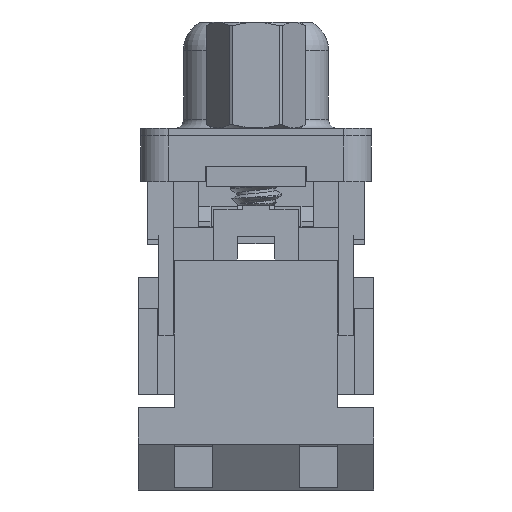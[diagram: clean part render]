
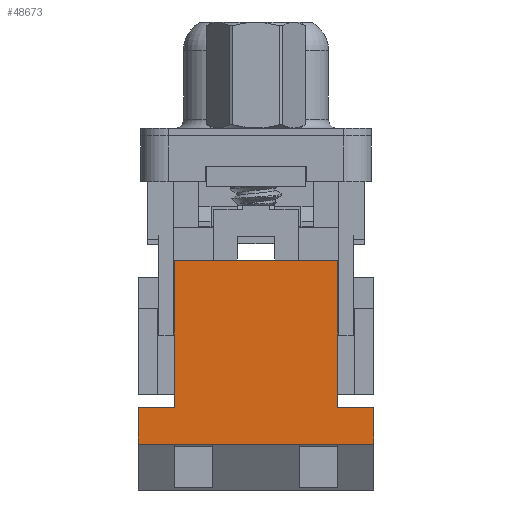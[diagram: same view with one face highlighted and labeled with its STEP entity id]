
A CAD part, left-side view. The second image highlights one B-rep face of the part: STEP entity #48673.
In plain terms, the highlighted planar face has unit normal (-1, 0, 0).
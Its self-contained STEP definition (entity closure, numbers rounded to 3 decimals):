
#1239 = EDGE_CURVE ( 'NONE', #46045, #82600, #1669, .T. ) ;
#1565 = LINE ( 'NONE', #59282, #43901 ) ;
#1669 = LINE ( 'NONE', #27736, #4810 ) ;
#4810 = VECTOR ( 'NONE', #8078, 1000. ) ;
#5013 = CARTESIAN_POINT ( 'NONE',  ( 3.245, 6.425, -14.8 ) ) ;
#7446 = ORIENTED_EDGE ( 'NONE', *, *, #13543, .F. ) ;
#7555 = DIRECTION ( 'NONE',  ( 0., -1., 0. ) ) ;
#8078 = DIRECTION ( 'NONE',  ( 0., 0., -1. ) ) ;
#9558 = EDGE_CURVE ( 'NONE', #14567, #82600, #25720, .T. ) ;
#10601 = CARTESIAN_POINT ( 'NONE',  ( 3.245, 4.45, -6.8 ) ) ;
#11469 = ORIENTED_EDGE ( 'NONE', *, *, #55813, .T. ) ;
#12076 = CARTESIAN_POINT ( 'NONE',  ( 3.245, -6.425, -16.8 ) ) ;
#13543 = EDGE_CURVE ( 'NONE', #46045, #62165, #39611, .T. ) ;
#14464 = CARTESIAN_POINT ( 'NONE',  ( 3.245, 6.425, -14.8 ) ) ;
#14567 = VERTEX_POINT ( 'NONE', #75580 ) ;
#16999 = LINE ( 'NONE', #43079, #81267 ) ;
#17155 = FACE_OUTER_BOUND ( 'NONE', #45554, .T. ) ;
#19388 = LINE ( 'NONE', #71533, #65400 ) ;
#20786 = EDGE_CURVE ( 'NONE', #35050, #14567, #19388, .T. ) ;
#21862 = PLANE ( 'NONE',  #29970 ) ;
#25720 = LINE ( 'NONE', #12076, #68399 ) ;
#27736 = CARTESIAN_POINT ( 'NONE',  ( 3.245, 6.425, -15.3 ) ) ;
#29970 = AXIS2_PLACEMENT_3D ( 'NONE', #43231, #67616, #69303 ) ;
#33811 = ORIENTED_EDGE ( 'NONE', *, *, #1239, .T. ) ;
#34139 = ORIENTED_EDGE ( 'NONE', *, *, #72278, .F. ) ;
#35050 = VERTEX_POINT ( 'NONE', #50139 ) ;
#39611 = LINE ( 'NONE', #78924, #49628 ) ;
#40540 = DIRECTION ( 'NONE',  ( 0., -1., 0. ) ) ;
#41027 = VERTEX_POINT ( 'NONE', #61676 ) ;
#41517 = CARTESIAN_POINT ( 'NONE',  ( 3.245, -4.45, -6.8 ) ) ;
#42377 = LINE ( 'NONE', #41517, #46023 ) ;
#43079 = CARTESIAN_POINT ( 'NONE',  ( 3.245, 4.45, -6.8 ) ) ;
#43231 = CARTESIAN_POINT ( 'NONE',  ( 3.245, -6.425, -15.3 ) ) ;
#43901 = VECTOR ( 'NONE', #52862, 1000. ) ;
#45554 = EDGE_LOOP ( 'NONE', ( #33811, #54687, #80344, #73086, #34139, #77305, #11469, #7446 ) ) ;
#46023 = VECTOR ( 'NONE', #67600, 1000. ) ;
#46045 = VERTEX_POINT ( 'NONE', #5013 ) ;
#48509 = VERTEX_POINT ( 'NONE', #73592 ) ;
#48673 = ADVANCED_FACE ( 'NONE', ( #17155 ), #21862, .F. ) ;
#49628 = VECTOR ( 'NONE', #7555, 1000. ) ;
#50139 = CARTESIAN_POINT ( 'NONE',  ( 3.245, -6.425, -14.8 ) ) ;
#52862 = DIRECTION ( 'NONE',  ( 0., -1., 0. ) ) ;
#54687 = ORIENTED_EDGE ( 'NONE', *, *, #9558, .F. ) ;
#55813 = EDGE_CURVE ( 'NONE', #59517, #62165, #16999, .T. ) ;
#59282 = CARTESIAN_POINT ( 'NONE',  ( 3.245, 4.45, -6.8 ) ) ;
#59517 = VERTEX_POINT ( 'NONE', #10601 ) ;
#59812 = CARTESIAN_POINT ( 'NONE',  ( 3.245, 4.45, -14.8 ) ) ;
#60031 = CARTESIAN_POINT ( 'NONE',  ( 3.245, 6.425, -16.8 ) ) ;
#61676 = CARTESIAN_POINT ( 'NONE',  ( 3.245, -4.45, -14.8 ) ) ;
#62165 = VERTEX_POINT ( 'NONE', #59812 ) ;
#65400 = VECTOR ( 'NONE', #65970, 1000. ) ;
#65970 = DIRECTION ( 'NONE',  ( 0., 0., -1. ) ) ;
#67600 = DIRECTION ( 'NONE',  ( 0., 0., -1. ) ) ;
#67616 = DIRECTION ( 'NONE',  ( 1., 0., 0. ) ) ;
#68399 = VECTOR ( 'NONE', #83031, 1000. ) ;
#68456 = EDGE_CURVE ( 'NONE', #41027, #35050, #73023, .T. ) ;
#69303 = DIRECTION ( 'NONE',  ( 0., 0., -1. ) ) ;
#71533 = CARTESIAN_POINT ( 'NONE',  ( 3.245, -6.425, -15.3 ) ) ;
#72278 = EDGE_CURVE ( 'NONE', #48509, #41027, #42377, .T. ) ;
#73023 = LINE ( 'NONE', #14464, #75566 ) ;
#73086 = ORIENTED_EDGE ( 'NONE', *, *, #68456, .F. ) ;
#73592 = CARTESIAN_POINT ( 'NONE',  ( 3.245, -4.45, -6.8 ) ) ;
#74713 = DIRECTION ( 'NONE',  ( 0., 0., -1. ) ) ;
#75566 = VECTOR ( 'NONE', #40540, 1000. ) ;
#75580 = CARTESIAN_POINT ( 'NONE',  ( 3.245, -6.425, -16.8 ) ) ;
#77305 = ORIENTED_EDGE ( 'NONE', *, *, #80923, .F. ) ;
#78924 = CARTESIAN_POINT ( 'NONE',  ( 3.245, 6.425, -14.8 ) ) ;
#80344 = ORIENTED_EDGE ( 'NONE', *, *, #20786, .F. ) ;
#80923 = EDGE_CURVE ( 'NONE', #59517, #48509, #1565, .T. ) ;
#81267 = VECTOR ( 'NONE', #74713, 1000. ) ;
#82600 = VERTEX_POINT ( 'NONE', #60031 ) ;
#83031 = DIRECTION ( 'NONE',  ( 0., 1., 0. ) ) ;
